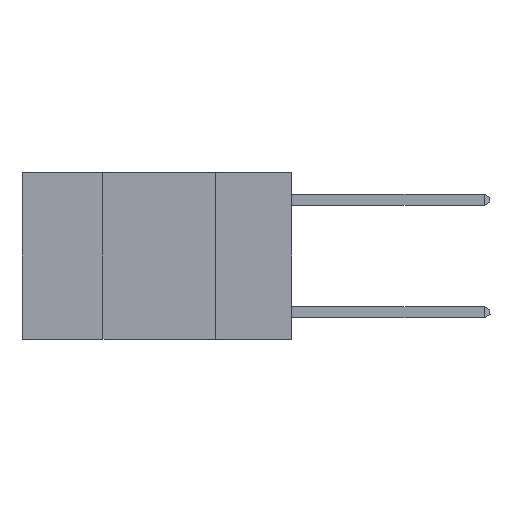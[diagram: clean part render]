
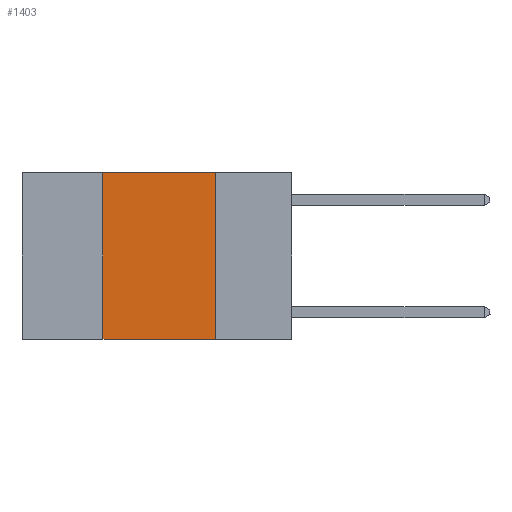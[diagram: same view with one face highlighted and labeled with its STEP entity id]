
A CAD part, left-side view. The second image highlights one B-rep face of the part: STEP entity #1403.
In plain terms, the highlighted planar face has unit normal (-1, 0, 0).
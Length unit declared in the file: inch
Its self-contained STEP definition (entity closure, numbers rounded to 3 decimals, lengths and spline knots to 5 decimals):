
#252 = CARTESIAN_POINT ( 'NONE',  ( 0., 0.42, 0. ) ) ;
#1403 = ADVANCED_FACE ( 'NONE', ( #1626 ), #22662, .F. ) ;
#1590 = VECTOR ( 'NONE', #2917, 39.37008 ) ;
#1626 = FACE_OUTER_BOUND ( 'NONE', #25788, .T. ) ;
#2308 = VECTOR ( 'NONE', #14880, 39.37008 ) ;
#2841 = CARTESIAN_POINT ( 'NONE',  ( 0., 0.6, 0. ) ) ;
#2917 = DIRECTION ( 'NONE',  ( 0., -1., 0. ) ) ;
#3107 = VERTEX_POINT ( 'NONE', #7111 ) ;
#3186 = CARTESIAN_POINT ( 'NONE',  ( 0., 0.6, -0.37 ) ) ;
#4682 = DIRECTION ( 'NONE',  ( 0., 0., -1. ) ) ;
#4939 = ORIENTED_EDGE ( 'NONE', *, *, #17365, .F. ) ;
#5239 = LINE ( 'NONE', #3186, #1590 ) ;
#6200 = EDGE_CURVE ( 'NONE', #3107, #18155, #19374, .T. ) ;
#7111 = CARTESIAN_POINT ( 'NONE',  ( 0., 0.42, 0. ) ) ;
#7457 = EDGE_CURVE ( 'NONE', #11127, #3107, #18420, .T. ) ;
#9007 = AXIS2_PLACEMENT_3D ( 'NONE', #12294, #20616, #16246 ) ;
#9576 = ORIENTED_EDGE ( 'NONE', *, *, #6200, .F. ) ;
#9650 = CARTESIAN_POINT ( 'NONE',  ( 0., 0.17, 0. ) ) ;
#11127 = VERTEX_POINT ( 'NONE', #12616 ) ;
#12294 = CARTESIAN_POINT ( 'NONE',  ( 0., 0.6, 0. ) ) ;
#12616 = CARTESIAN_POINT ( 'NONE',  ( 0., 0.42, -0.37 ) ) ;
#13166 = LINE ( 'NONE', #23941, #16511 ) ;
#13812 = EDGE_CURVE ( 'NONE', #11127, #17697, #5239, .T. ) ;
#14363 = CARTESIAN_POINT ( 'NONE',  ( 0., 0.17, -0.37 ) ) ;
#14608 = DIRECTION ( 'NONE',  ( 0., 0., 1. ) ) ;
#14880 = DIRECTION ( 'NONE',  ( 0., -1., 0. ) ) ;
#16246 = DIRECTION ( 'NONE',  ( 0., 0., -1. ) ) ;
#16511 = VECTOR ( 'NONE', #4682, 39.37008 ) ;
#17365 = EDGE_CURVE ( 'NONE', #18155, #17697, #13166, .T. ) ;
#17697 = VERTEX_POINT ( 'NONE', #14363 ) ;
#18155 = VERTEX_POINT ( 'NONE', #9650 ) ;
#18251 = ORIENTED_EDGE ( 'NONE', *, *, #13812, .T. ) ;
#18420 = LINE ( 'NONE', #252, #23662 ) ;
#19374 = LINE ( 'NONE', #2841, #2308 ) ;
#20616 = DIRECTION ( 'NONE',  ( 1., 0., 0. ) ) ;
#22662 = PLANE ( 'NONE',  #9007 ) ;
#23171 = ORIENTED_EDGE ( 'NONE', *, *, #7457, .F. ) ;
#23662 = VECTOR ( 'NONE', #14608, 39.37008 ) ;
#23941 = CARTESIAN_POINT ( 'NONE',  ( 0., 0.17, 0. ) ) ;
#25788 = EDGE_LOOP ( 'NONE', ( #4939, #9576, #23171, #18251 ) ) ;
